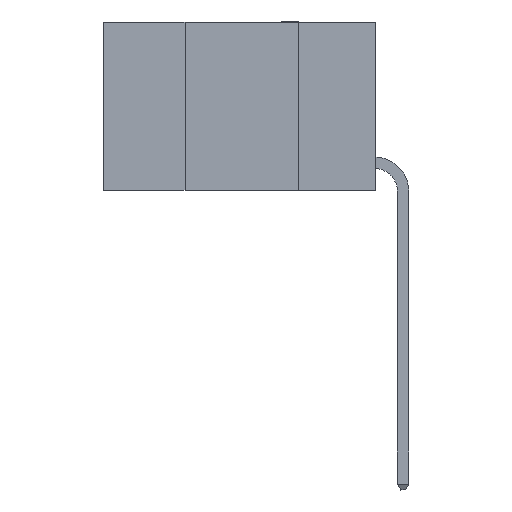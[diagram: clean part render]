
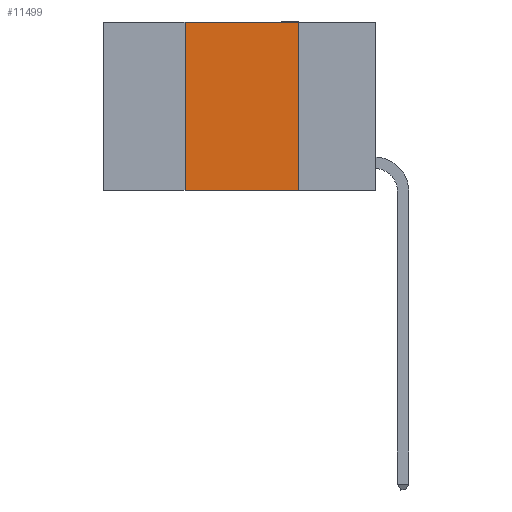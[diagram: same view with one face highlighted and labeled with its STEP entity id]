
A CAD part, left-side view. The second image highlights one B-rep face of the part: STEP entity #11499.
In plain terms, the highlighted planar face has unit normal (-1, 0, 0).
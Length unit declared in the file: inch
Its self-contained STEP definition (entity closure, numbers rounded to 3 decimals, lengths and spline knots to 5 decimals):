
#236 = VECTOR ( 'NONE', #2895, 39.37008 ) ;
#408 = CARTESIAN_POINT ( 'NONE',  ( 0., 0.42, 0. ) ) ;
#1173 = LINE ( 'NONE', #11547, #4647 ) ;
#1787 = CARTESIAN_POINT ( 'NONE',  ( 0., 0.17, 0. ) ) ;
#1788 = CARTESIAN_POINT ( 'NONE',  ( 0., 0.17, -0.37 ) ) ;
#1796 = EDGE_LOOP ( 'NONE', ( #5708, #2716, #5405, #8035 ) ) ;
#2175 = CARTESIAN_POINT ( 'NONE',  ( 0., 0.6, 0. ) ) ;
#2496 = AXIS2_PLACEMENT_3D ( 'NONE', #2175, #6015, #7648 ) ;
#2716 = ORIENTED_EDGE ( 'NONE', *, *, #4266, .F. ) ;
#2895 = DIRECTION ( 'NONE',  ( 0., 0., -1. ) ) ;
#4266 = EDGE_CURVE ( 'NONE', #11394, #10082, #10894, .T. ) ;
#4647 = VECTOR ( 'NONE', #8544, 39.37008 ) ;
#5262 = DIRECTION ( 'NONE',  ( 0., -1., 0. ) ) ;
#5405 = ORIENTED_EDGE ( 'NONE', *, *, #10220, .F. ) ;
#5708 = ORIENTED_EDGE ( 'NONE', *, *, #5886, .F. ) ;
#5766 = PLANE ( 'NONE',  #2496 ) ;
#5779 = VERTEX_POINT ( 'NONE', #1788 ) ;
#5819 = VECTOR ( 'NONE', #5262, 39.37008 ) ;
#5886 = EDGE_CURVE ( 'NONE', #10082, #5779, #9597, .T. ) ;
#6015 = DIRECTION ( 'NONE',  ( 1., 0., 0. ) ) ;
#6555 = VERTEX_POINT ( 'NONE', #11896 ) ;
#6783 = LINE ( 'NONE', #9915, #5819 ) ;
#7648 = DIRECTION ( 'NONE',  ( 0., 0., -1. ) ) ;
#8035 = ORIENTED_EDGE ( 'NONE', *, *, #9901, .T. ) ;
#8093 = VECTOR ( 'NONE', #11683, 39.37008 ) ;
#8544 = DIRECTION ( 'NONE',  ( 0., 0., 1. ) ) ;
#8580 = FACE_OUTER_BOUND ( 'NONE', #1796, .T. ) ;
#9597 = LINE ( 'NONE', #10328, #236 ) ;
#9901 = EDGE_CURVE ( 'NONE', #6555, #5779, #6783, .T. ) ;
#9915 = CARTESIAN_POINT ( 'NONE',  ( 0., 0.6, -0.37 ) ) ;
#10082 = VERTEX_POINT ( 'NONE', #1787 ) ;
#10220 = EDGE_CURVE ( 'NONE', #6555, #11394, #1173, .T. ) ;
#10328 = CARTESIAN_POINT ( 'NONE',  ( 0., 0.17, 0. ) ) ;
#10715 = CARTESIAN_POINT ( 'NONE',  ( 0., 0.6, 0. ) ) ;
#10894 = LINE ( 'NONE', #10715, #8093 ) ;
#11394 = VERTEX_POINT ( 'NONE', #408 ) ;
#11499 = ADVANCED_FACE ( 'NONE', ( #8580 ), #5766, .F. ) ;
#11547 = CARTESIAN_POINT ( 'NONE',  ( 0., 0.42, 0. ) ) ;
#11683 = DIRECTION ( 'NONE',  ( 0., -1., 0. ) ) ;
#11896 = CARTESIAN_POINT ( 'NONE',  ( 0., 0.42, -0.37 ) ) ;
